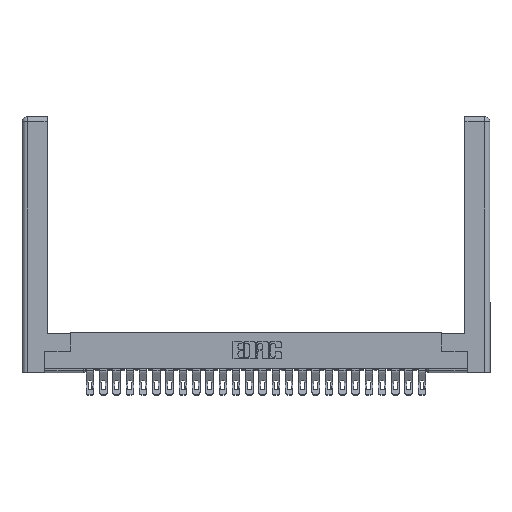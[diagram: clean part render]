
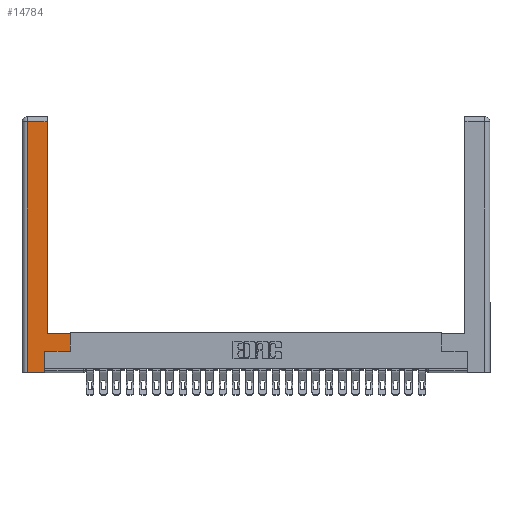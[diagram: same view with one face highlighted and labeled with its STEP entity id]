
A CAD part, top view. The second image highlights one B-rep face of the part: STEP entity #14784.
In plain terms, the highlighted planar face has unit normal (0, 0, 1).
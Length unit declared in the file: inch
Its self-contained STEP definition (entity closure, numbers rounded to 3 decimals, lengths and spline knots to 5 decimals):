
#230 = CARTESIAN_POINT ( 'NONE',  ( 0., 0., 0. ) ) ;
#974 = VECTOR ( 'NONE', #11666, 39.37008 ) ;
#1656 = ORIENTED_EDGE ( 'NONE', *, *, #28033, .T. ) ;
#1719 = LINE ( 'NONE', #25327, #18426 ) ;
#1979 = EDGE_CURVE ( 'NONE', #17309, #6978, #4521, .T. ) ;
#2435 = DIRECTION ( 'NONE',  ( -1., 0., 0. ) ) ;
#3079 = EDGE_CURVE ( 'NONE', #10428, #17309, #27999, .T. ) ;
#3087 = VECTOR ( 'NONE', #22802, 39.37008 ) ;
#3586 = DIRECTION ( 'NONE',  ( 0., 1., 0. ) ) ;
#4521 = LINE ( 'NONE', #26553, #11651 ) ;
#4695 = VECTOR ( 'NONE', #3586, 39.37008 ) ;
#4726 = CARTESIAN_POINT ( 'NONE',  ( 0.0615, 0., 0. ) ) ;
#4815 = VERTEX_POINT ( 'NONE', #4726 ) ;
#5177 = EDGE_LOOP ( 'NONE', ( #14933, #6402, #12906, #27879, #1656, #20046, #24917, #22981 ) ) ;
#5406 = FACE_OUTER_BOUND ( 'NONE', #5177, .T. ) ;
#5817 = EDGE_CURVE ( 'NONE', #9887, #27597, #23779, .T. ) ;
#6140 = DIRECTION ( 'NONE',  ( -1., 0., 0. ) ) ;
#6282 = CARTESIAN_POINT ( 'NONE',  ( 0.0615, 2.94, 0. ) ) ;
#6402 = ORIENTED_EDGE ( 'NONE', *, *, #5817, .T. ) ;
#6833 = EDGE_CURVE ( 'NONE', #27597, #4815, #1719, .T. ) ;
#6873 = DIRECTION ( 'NONE',  ( 1., 0., 0. ) ) ;
#6978 = VERTEX_POINT ( 'NONE', #10370 ) ;
#7037 = CARTESIAN_POINT ( 'NONE',  ( 0.295, 0.45, 0. ) ) ;
#7555 = CARTESIAN_POINT ( 'NONE',  ( 0.565, 0.245, 0. ) ) ;
#7943 = EDGE_CURVE ( 'NONE', #6978, #10926, #12567, .T. ) ;
#8720 = DIRECTION ( 'NONE',  ( 0., 1., 0. ) ) ;
#8775 = CARTESIAN_POINT ( 'NONE',  ( 0.565, 0.245, 0. ) ) ;
#9887 = VERTEX_POINT ( 'NONE', #13316 ) ;
#10141 = VECTOR ( 'NONE', #8720, 39.37008 ) ;
#10370 = CARTESIAN_POINT ( 'NONE',  ( 0.565, 0.45, 0. ) ) ;
#10428 = VERTEX_POINT ( 'NONE', #18308 ) ;
#10813 = CARTESIAN_POINT ( 'NONE',  ( 0.265, 0.245, 0. ) ) ;
#10926 = VERTEX_POINT ( 'NONE', #7037 ) ;
#11056 = AXIS2_PLACEMENT_3D ( 'NONE', #230, #22273, #2435 ) ;
#11651 = VECTOR ( 'NONE', #24430, 39.37008 ) ;
#11666 = DIRECTION ( 'NONE',  ( -1., 0., 0. ) ) ;
#12125 = DIRECTION ( 'NONE',  ( 0., -1., 0. ) ) ;
#12567 = LINE ( 'NONE', #26875, #974 ) ;
#12906 = ORIENTED_EDGE ( 'NONE', *, *, #6833, .T. ) ;
#13316 = CARTESIAN_POINT ( 'NONE',  ( 0.295, 2.94, 0. ) ) ;
#13618 = VECTOR ( 'NONE', #6873, 39.37008 ) ;
#14784 = ADVANCED_FACE ( 'NONE', ( #5406 ), #26400, .F. ) ;
#14933 = ORIENTED_EDGE ( 'NONE', *, *, #27936, .T. ) ;
#17309 = VERTEX_POINT ( 'NONE', #8775 ) ;
#17626 = CARTESIAN_POINT ( 'NONE',  ( 0.265, 0., 0. ) ) ;
#18308 = CARTESIAN_POINT ( 'NONE',  ( 0.265, 0.245, 0. ) ) ;
#18426 = VECTOR ( 'NONE', #12125, 39.37008 ) ;
#19334 = LINE ( 'NONE', #10813, #10141 ) ;
#19417 = LINE ( 'NONE', #17626, #13618 ) ;
#20019 = VECTOR ( 'NONE', #6140, 39.37008 ) ;
#20046 = ORIENTED_EDGE ( 'NONE', *, *, #3079, .T. ) ;
#22273 = DIRECTION ( 'NONE',  ( 0., 0., -1. ) ) ;
#22802 = DIRECTION ( 'NONE',  ( 1., 0., 0. ) ) ;
#22981 = ORIENTED_EDGE ( 'NONE', *, *, #7943, .T. ) ;
#23125 = CARTESIAN_POINT ( 'NONE',  ( 0.295, 3., 0. ) ) ;
#23132 = LINE ( 'NONE', #23125, #4695 ) ;
#23779 = LINE ( 'NONE', #28172, #20019 ) ;
#24430 = DIRECTION ( 'NONE',  ( 0., 1., 0. ) ) ;
#24917 = ORIENTED_EDGE ( 'NONE', *, *, #1979, .T. ) ;
#25006 = VERTEX_POINT ( 'NONE', #25791 ) ;
#25023 = EDGE_CURVE ( 'NONE', #4815, #25006, #19417, .T. ) ;
#25327 = CARTESIAN_POINT ( 'NONE',  ( 0.0615, 0., 0. ) ) ;
#25791 = CARTESIAN_POINT ( 'NONE',  ( 0.265, 0., 0. ) ) ;
#26400 = PLANE ( 'NONE',  #11056 ) ;
#26553 = CARTESIAN_POINT ( 'NONE',  ( 0.565, 0.45, 0. ) ) ;
#26875 = CARTESIAN_POINT ( 'NONE',  ( 0.295, 0.45, 0. ) ) ;
#27597 = VERTEX_POINT ( 'NONE', #6282 ) ;
#27879 = ORIENTED_EDGE ( 'NONE', *, *, #25023, .T. ) ;
#27936 = EDGE_CURVE ( 'NONE', #10926, #9887, #23132, .T. ) ;
#27999 = LINE ( 'NONE', #7555, #3087 ) ;
#28033 = EDGE_CURVE ( 'NONE', #25006, #10428, #19334, .T. ) ;
#28172 = CARTESIAN_POINT ( 'NONE',  ( 0.0615, 2.94, 0. ) ) ;
